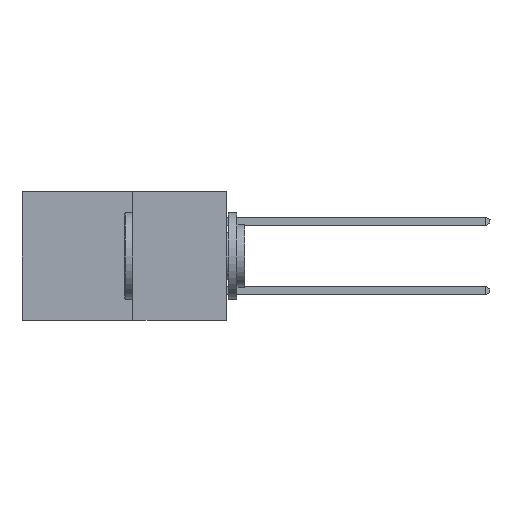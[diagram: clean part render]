
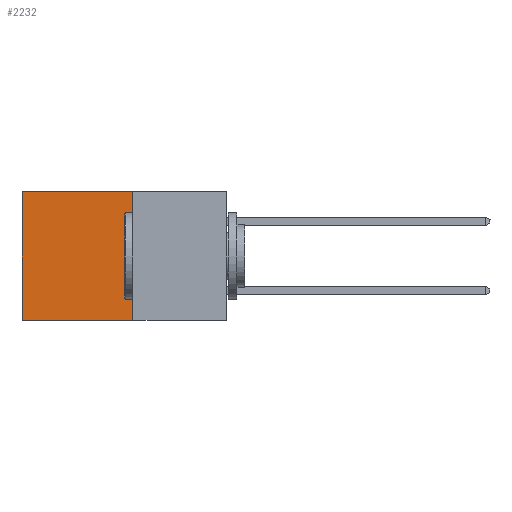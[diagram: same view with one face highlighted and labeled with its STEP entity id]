
A CAD part, left-side view. The second image highlights one B-rep face of the part: STEP entity #2232.
In plain terms, the highlighted planar face has unit normal (-1, 0, 0).
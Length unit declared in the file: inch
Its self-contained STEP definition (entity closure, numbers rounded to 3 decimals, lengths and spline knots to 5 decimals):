
#41 = LINE ( 'NONE', #2852, #4546 ) ;
#334 = CARTESIAN_POINT ( 'NONE',  ( 0.277, 0.27, 0. ) ) ;
#849 = PLANE ( 'NONE',  #12679 ) ;
#1780 = DIRECTION ( 'NONE',  ( 0., 0., -1. ) ) ;
#2232 = ADVANCED_FACE ( 'NONE', ( #11613 ), #849, .F. ) ;
#2284 = EDGE_CURVE ( 'NONE', #17618, #8912, #41, .T. ) ;
#2369 = EDGE_CURVE ( 'NONE', #17957, #16525, #25794, .T. ) ;
#2444 = CARTESIAN_POINT ( 'NONE',  ( 0.277, 0.59, -0.37 ) ) ;
#2852 = CARTESIAN_POINT ( 'NONE',  ( 0.277, 0.27, -0.37 ) ) ;
#4546 = VECTOR ( 'NONE', #26215, 39.37008 ) ;
#6031 = CARTESIAN_POINT ( 'NONE',  ( 0.277, 0.59, -0.37 ) ) ;
#6126 = DIRECTION ( 'NONE',  ( 0., 0., -1. ) ) ;
#6318 = CARTESIAN_POINT ( 'NONE',  ( 0.277, 0.27, 0. ) ) ;
#7541 = ORIENTED_EDGE ( 'NONE', *, *, #2369, .T. ) ;
#8912 = VERTEX_POINT ( 'NONE', #2444 ) ;
#10323 = CARTESIAN_POINT ( 'NONE',  ( 0.277, 0.27, -0.37 ) ) ;
#10499 = EDGE_CURVE ( 'NONE', #16525, #8912, #27374, .T. ) ;
#11613 = FACE_OUTER_BOUND ( 'NONE', #27219, .T. ) ;
#12679 = AXIS2_PLACEMENT_3D ( 'NONE', #10323, #15232, #18087 ) ;
#13233 = CARTESIAN_POINT ( 'NONE',  ( 0.277, 0.59, 0. ) ) ;
#14851 = LINE ( 'NONE', #27268, #19149 ) ;
#15232 = DIRECTION ( 'NONE',  ( 1., 0., 0. ) ) ;
#16525 = VERTEX_POINT ( 'NONE', #13233 ) ;
#17269 = ORIENTED_EDGE ( 'NONE', *, *, #17760, .F. ) ;
#17618 = VERTEX_POINT ( 'NONE', #22747 ) ;
#17760 = EDGE_CURVE ( 'NONE', #17957, #17618, #14851, .T. ) ;
#17957 = VERTEX_POINT ( 'NONE', #334 ) ;
#18087 = DIRECTION ( 'NONE',  ( 0., 0., -1. ) ) ;
#18259 = VECTOR ( 'NONE', #6126, 39.37008 ) ;
#19149 = VECTOR ( 'NONE', #1780, 39.37008 ) ;
#22747 = CARTESIAN_POINT ( 'NONE',  ( 0.277, 0.27, -0.37 ) ) ;
#24672 = ORIENTED_EDGE ( 'NONE', *, *, #2284, .F. ) ;
#25121 = VECTOR ( 'NONE', #25444, 39.37008 ) ;
#25444 = DIRECTION ( 'NONE',  ( 0., 1., 0. ) ) ;
#25794 = LINE ( 'NONE', #6318, #25121 ) ;
#26215 = DIRECTION ( 'NONE',  ( 0., 1., 0. ) ) ;
#26874 = ORIENTED_EDGE ( 'NONE', *, *, #10499, .T. ) ;
#27219 = EDGE_LOOP ( 'NONE', ( #26874, #24672, #17269, #7541 ) ) ;
#27268 = CARTESIAN_POINT ( 'NONE',  ( 0.277, 0.27, -0.37 ) ) ;
#27374 = LINE ( 'NONE', #6031, #18259 ) ;
